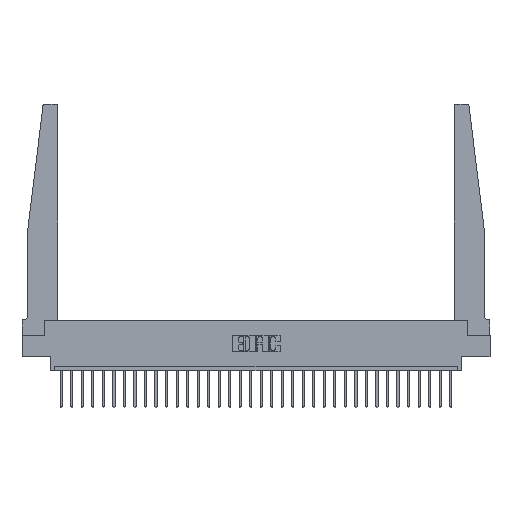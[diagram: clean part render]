
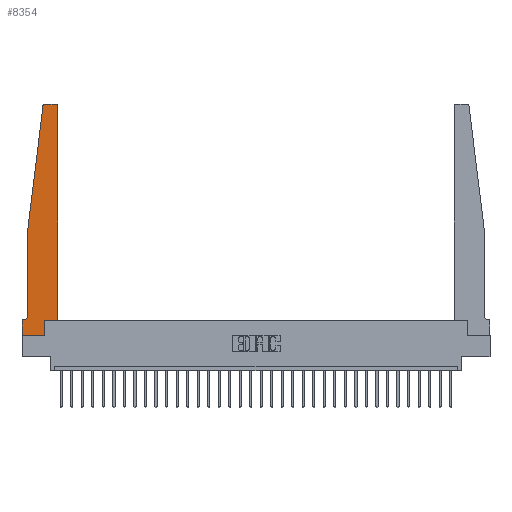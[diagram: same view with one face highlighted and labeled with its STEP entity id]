
A CAD part, top view. The second image highlights one B-rep face of the part: STEP entity #8354.
In plain terms, the highlighted planar face has unit normal (0, 0, 1).
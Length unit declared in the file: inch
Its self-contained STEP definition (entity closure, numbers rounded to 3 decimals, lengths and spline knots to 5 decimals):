
#737 = CARTESIAN_POINT ( 'NONE',  ( 0.065, 0.2375, 0.37 ) ) ;
#1174 = VERTEX_POINT ( 'NONE', #9120 ) ;
#1319 = EDGE_CURVE ( 'NONE', #12113, #19022, #22432, .T. ) ;
#1560 = CARTESIAN_POINT ( 'NONE',  ( 0.2605, 0.18, 0.37 ) ) ;
#1621 = VECTOR ( 'NONE', #26920, 39.37008 ) ;
#2184 = VECTOR ( 'NONE', #17691, 39.37008 ) ;
#2432 = DIRECTION ( 'NONE',  ( -1., 0., 0. ) ) ;
#2492 = ORIENTED_EDGE ( 'NONE', *, *, #19872, .T. ) ;
#2908 = EDGE_CURVE ( 'NONE', #12388, #15058, #24435, .T. ) ;
#3305 = DIRECTION ( 'NONE',  ( 1., 0., 0. ) ) ;
#3333 = EDGE_CURVE ( 'NONE', #19022, #27485, #19887, .T. ) ;
#3918 = DIRECTION ( 'NONE',  ( 0., -1., 0. ) ) ;
#4123 = ORIENTED_EDGE ( 'NONE', *, *, #21953, .T. ) ;
#4124 = CARTESIAN_POINT ( 'NONE',  ( 0.065, 1.25, 0.37 ) ) ;
#4645 = LINE ( 'NONE', #1560, #2184 ) ;
#5155 = ORIENTED_EDGE ( 'NONE', *, *, #28736, .T. ) ;
#5334 = CARTESIAN_POINT ( 'NONE',  ( 0.27653, 2.72, 0.37 ) ) ;
#5342 = ORIENTED_EDGE ( 'NONE', *, *, #10746, .T. ) ;
#5688 = VERTEX_POINT ( 'NONE', #19370 ) ;
#6241 = ORIENTED_EDGE ( 'NONE', *, *, #17584, .T. ) ;
#6659 = CARTESIAN_POINT ( 'NONE',  ( 0.24675, 2.72367, 0.37 ) ) ;
#6957 = AXIS2_PLACEMENT_3D ( 'NONE', #16321, #22907, #25742 ) ;
#6959 = CARTESIAN_POINT ( 'NONE',  ( 0.425, 2.72, 0.37 ) ) ;
#7310 = DIRECTION ( 'NONE',  ( 1., 0., 0. ) ) ;
#7328 = VECTOR ( 'NONE', #3918, 39.37008 ) ;
#7713 = LINE ( 'NONE', #9779, #12295 ) ;
#8145 = VERTEX_POINT ( 'NONE', #6959 ) ;
#8354 = ADVANCED_FACE ( 'NONE', ( #9932 ), #21173, .T. ) ;
#8610 = VERTEX_POINT ( 'NONE', #21854 ) ;
#8776 = CIRCLE ( 'NONE', #19183, 0.05 ) ;
#8842 = DIRECTION ( 'NONE',  ( 0., 0., 1. ) ) ;
#9120 = CARTESIAN_POINT ( 'NONE',  ( 0.27653, 2.75, 0.37 ) ) ;
#9524 = EDGE_CURVE ( 'NONE', #1174, #12113, #11982, .T. ) ;
#9569 = CARTESIAN_POINT ( 'NONE',  ( 0.065, 1.25, 0.37 ) ) ;
#9779 = CARTESIAN_POINT ( 'NONE',  ( 0., 0., 0.37 ) ) ;
#9785 = CARTESIAN_POINT ( 'NONE',  ( 0.25, 2.75, 0.37 ) ) ;
#9816 = AXIS2_PLACEMENT_3D ( 'NONE', #10735, #8842, #24491 ) ;
#9932 = FACE_OUTER_BOUND ( 'NONE', #25938, .T. ) ;
#10256 = EDGE_CURVE ( 'NONE', #22952, #5688, #7713, .T. ) ;
#10517 = LINE ( 'NONE', #15370, #7328 ) ;
#10707 = DIRECTION ( 'NONE',  ( -1., 0., 0. ) ) ;
#10735 = CARTESIAN_POINT ( 'NONE',  ( 0.395, 2.72, 0.37 ) ) ;
#10746 = EDGE_CURVE ( 'NONE', #15058, #22952, #10517, .T. ) ;
#11982 = CIRCLE ( 'NONE', #28366, 0.03 ) ;
#12113 = VERTEX_POINT ( 'NONE', #6659 ) ;
#12260 = LINE ( 'NONE', #26780, #17892 ) ;
#12295 = VECTOR ( 'NONE', #7310, 39.37008 ) ;
#12388 = VERTEX_POINT ( 'NONE', #23533 ) ;
#12431 = LINE ( 'NONE', #9785, #18091 ) ;
#15058 = VERTEX_POINT ( 'NONE', #17117 ) ;
#15370 = CARTESIAN_POINT ( 'NONE',  ( 0., 0., 0.37 ) ) ;
#15428 = ORIENTED_EDGE ( 'NONE', *, *, #25363, .T. ) ;
#15963 = ORIENTED_EDGE ( 'NONE', *, *, #9524, .T. ) ;
#16089 = ORIENTED_EDGE ( 'NONE', *, *, #1319, .T. ) ;
#16097 = VECTOR ( 'NONE', #2432, 39.37008 ) ;
#16247 = CARTESIAN_POINT ( 'NONE',  ( 0.2605, 0.18, 0.37 ) ) ;
#16321 = CARTESIAN_POINT ( 'NONE',  ( 0., 0.1875, 0.37 ) ) ;
#16701 = DIRECTION ( 'NONE',  ( 0., 0., 1. ) ) ;
#16917 = DIRECTION ( 'NONE',  ( 0., 0., -1. ) ) ;
#17117 = CARTESIAN_POINT ( 'NONE',  ( 0., 0.1875, 0.37 ) ) ;
#17584 = EDGE_CURVE ( 'NONE', #24096, #1174, #12431, .T. ) ;
#17691 = DIRECTION ( 'NONE',  ( 0., 1., 0. ) ) ;
#17892 = VECTOR ( 'NONE', #26870, 39.37008 ) ;
#18091 = VECTOR ( 'NONE', #18446, 39.37008 ) ;
#18446 = DIRECTION ( 'NONE',  ( -1., 0., 0. ) ) ;
#18677 = LINE ( 'NONE', #20419, #21798 ) ;
#19022 = VERTEX_POINT ( 'NONE', #4124 ) ;
#19183 = AXIS2_PLACEMENT_3D ( 'NONE', #24661, #16917, #10707 ) ;
#19370 = CARTESIAN_POINT ( 'NONE',  ( 0.2605, 0., 0.37 ) ) ;
#19872 = EDGE_CURVE ( 'NONE', #27485, #12388, #8776, .T. ) ;
#19887 = LINE ( 'NONE', #22726, #1621 ) ;
#20023 = VECTOR ( 'NONE', #26072, 39.37008 ) ;
#20340 = EDGE_CURVE ( 'NONE', #20999, #8610, #12260, .T. ) ;
#20419 = CARTESIAN_POINT ( 'NONE',  ( 0.425, 0.18, 0.37 ) ) ;
#20573 = CARTESIAN_POINT ( 'NONE',  ( 0.395, 2.75, 0.37 ) ) ;
#20999 = VERTEX_POINT ( 'NONE', #16247 ) ;
#21173 = PLANE ( 'NONE',  #6957 ) ;
#21798 = VECTOR ( 'NONE', #25100, 39.37008 ) ;
#21854 = CARTESIAN_POINT ( 'NONE',  ( 0.425, 0.18, 0.37 ) ) ;
#21953 = EDGE_CURVE ( 'NONE', #8145, #24096, #28580, .T. ) ;
#22164 = ORIENTED_EDGE ( 'NONE', *, *, #10256, .T. ) ;
#22432 = LINE ( 'NONE', #9569, #20023 ) ;
#22662 = ORIENTED_EDGE ( 'NONE', *, *, #3333, .T. ) ;
#22677 = CARTESIAN_POINT ( 'NONE',  ( 0., 0., 0.37 ) ) ;
#22726 = CARTESIAN_POINT ( 'NONE',  ( 0.065, 1.25, 0.37 ) ) ;
#22907 = DIRECTION ( 'NONE',  ( 0., 0., 1. ) ) ;
#22952 = VERTEX_POINT ( 'NONE', #22677 ) ;
#23533 = CARTESIAN_POINT ( 'NONE',  ( 0.015, 0.1875, 0.37 ) ) ;
#24096 = VERTEX_POINT ( 'NONE', #20573 ) ;
#24435 = LINE ( 'NONE', #24888, #16097 ) ;
#24491 = DIRECTION ( 'NONE',  ( 1., 0., 0. ) ) ;
#24661 = CARTESIAN_POINT ( 'NONE',  ( 0.015, 0.2375, 0.37 ) ) ;
#24830 = ORIENTED_EDGE ( 'NONE', *, *, #20340, .T. ) ;
#24888 = CARTESIAN_POINT ( 'NONE',  ( 0.065, 0.1875, 0.37 ) ) ;
#25100 = DIRECTION ( 'NONE',  ( 0., 1., 0. ) ) ;
#25363 = EDGE_CURVE ( 'NONE', #8610, #8145, #18677, .T. ) ;
#25742 = DIRECTION ( 'NONE',  ( 1., 0., 0. ) ) ;
#25884 = ORIENTED_EDGE ( 'NONE', *, *, #2908, .T. ) ;
#25938 = EDGE_LOOP ( 'NONE', ( #6241, #15963, #16089, #22662, #2492, #25884, #5342, #22164, #5155, #24830, #15428, #4123 ) ) ;
#26072 = DIRECTION ( 'NONE',  ( -0.122, -0.992, 0. ) ) ;
#26780 = CARTESIAN_POINT ( 'NONE',  ( 0.425, 0.18, 0.37 ) ) ;
#26870 = DIRECTION ( 'NONE',  ( 1., 0., 0. ) ) ;
#26920 = DIRECTION ( 'NONE',  ( 0., -1., 0. ) ) ;
#27485 = VERTEX_POINT ( 'NONE', #737 ) ;
#28366 = AXIS2_PLACEMENT_3D ( 'NONE', #5334, #16701, #3305 ) ;
#28580 = CIRCLE ( 'NONE', #9816, 0.03 ) ;
#28736 = EDGE_CURVE ( 'NONE', #5688, #20999, #4645, .T. ) ;
